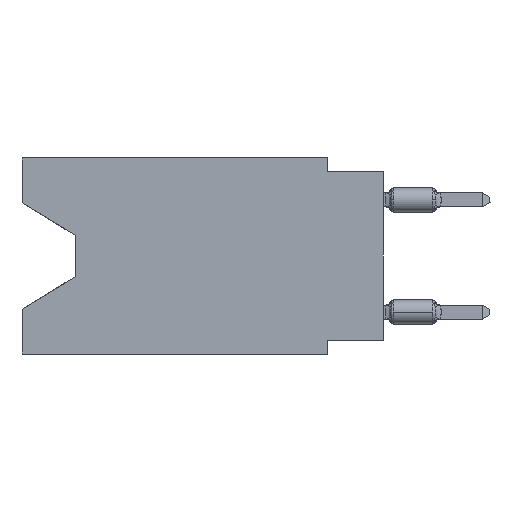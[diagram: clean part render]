
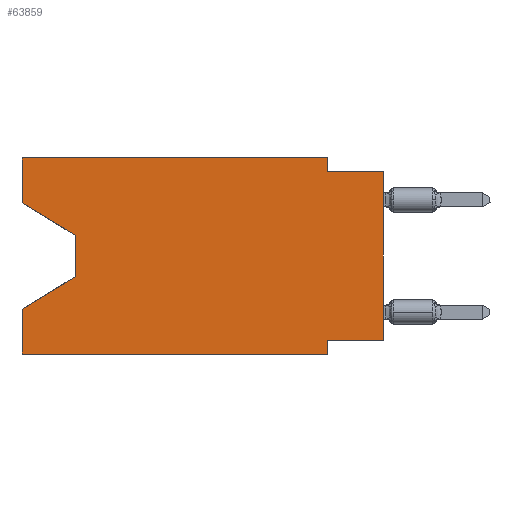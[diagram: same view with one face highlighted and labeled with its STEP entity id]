
A CAD part, left-side view. The second image highlights one B-rep face of the part: STEP entity #63859.
In plain terms, the highlighted planar face has unit normal (-1, 0, 0).
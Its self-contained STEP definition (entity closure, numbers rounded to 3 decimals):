
#559 = CARTESIAN_POINT ( 'NONE',  ( 0., 16.383, 0. ) ) ;
#798 = DIRECTION ( 'NONE',  ( 0., 1., 0. ) ) ;
#1833 = CARTESIAN_POINT ( 'NONE',  ( 0., 16.383, -8.89 ) ) ;
#2455 = VERTEX_POINT ( 'NONE', #49989 ) ;
#4818 = EDGE_CURVE ( 'NONE', #67629, #2455, #16789, .T. ) ;
#5903 = VECTOR ( 'NONE', #16608, 1000. ) ;
#6287 = VECTOR ( 'NONE', #33199, 1000. ) ;
#6741 = EDGE_CURVE ( 'NONE', #42762, #55426, #18316, .T. ) ;
#9593 = LINE ( 'NONE', #45181, #66337 ) ;
#9810 = DIRECTION ( 'NONE',  ( 0., -1., 0. ) ) ;
#10538 = VERTEX_POINT ( 'NONE', #1833 ) ;
#10824 = LINE ( 'NONE', #31768, #51969 ) ;
#13276 = CARTESIAN_POINT ( 'NONE',  ( 0., 16.383, -2.038 ) ) ;
#13336 = VECTOR ( 'NONE', #17821, 1000. ) ;
#13357 = ORIENTED_EDGE ( 'NONE', *, *, #4818, .T. ) ;
#13374 = LINE ( 'NONE', #45108, #52631 ) ;
#13657 = EDGE_LOOP ( 'NONE', ( #64866, #23779, #13357, #47135, #57510, #18241, #57631, #34532, #55323, #53581, #33526, #62559 ) ) ;
#16271 = CARTESIAN_POINT ( 'NONE',  ( 0., 13.97, -3.505 ) ) ;
#16608 = DIRECTION ( 'NONE',  ( 0., 0., 1. ) ) ;
#16789 = LINE ( 'NONE', #22018, #13336 ) ;
#17290 = CARTESIAN_POINT ( 'NONE',  ( 0., 13.97, -5.385 ) ) ;
#17821 = DIRECTION ( 'NONE',  ( 0., 0.855, -0.519 ) ) ;
#18241 = ORIENTED_EDGE ( 'NONE', *, *, #68927, .F. ) ;
#18316 = LINE ( 'NONE', #38890, #57024 ) ;
#18526 = LINE ( 'NONE', #13276, #6287 ) ;
#18632 = DIRECTION ( 'NONE',  ( 0., 0., -1. ) ) ;
#19743 = LINE ( 'NONE', #36111, #25132 ) ;
#20969 = DIRECTION ( 'NONE',  ( 0., 0., 1. ) ) ;
#21342 = LINE ( 'NONE', #42579, #40229 ) ;
#22018 = CARTESIAN_POINT ( 'NONE',  ( 0., 13.97, -5.385 ) ) ;
#23779 = ORIENTED_EDGE ( 'NONE', *, *, #60711, .T. ) ;
#23860 = DIRECTION ( 'NONE',  ( 0., -1., 0. ) ) ;
#24465 = VERTEX_POINT ( 'NONE', #47426 ) ;
#24531 = LINE ( 'NONE', #29422, #46024 ) ;
#25132 = VECTOR ( 'NONE', #45865, 1000. ) ;
#25624 = EDGE_CURVE ( 'NONE', #47585, #42762, #10824, .T. ) ;
#26387 = VERTEX_POINT ( 'NONE', #26996 ) ;
#26996 = CARTESIAN_POINT ( 'NONE',  ( 0., 2.54, -8.255 ) ) ;
#29287 = EDGE_CURVE ( 'NONE', #10538, #54925, #19743, .T. ) ;
#29293 = EDGE_CURVE ( 'NONE', #24465, #31701, #9593, .T. ) ;
#29422 = CARTESIAN_POINT ( 'NONE',  ( 0., 2.54, 0. ) ) ;
#30089 = EDGE_CURVE ( 'NONE', #47585, #36011, #18526, .T. ) ;
#30134 = DIRECTION ( 'NONE',  ( 0., 0., -1. ) ) ;
#30615 = DIRECTION ( 'NONE',  ( 1., 0., 0. ) ) ;
#31701 = VERTEX_POINT ( 'NONE', #54709 ) ;
#31768 = CARTESIAN_POINT ( 'NONE',  ( 0., 16.383, 0. ) ) ;
#32199 = CARTESIAN_POINT ( 'NONE',  ( 0., 0., -8.255 ) ) ;
#33199 = DIRECTION ( 'NONE',  ( 0., -0.855, -0.519 ) ) ;
#33526 = ORIENTED_EDGE ( 'NONE', *, *, #6741, .F. ) ;
#34532 = ORIENTED_EDGE ( 'NONE', *, *, #29293, .T. ) ;
#36011 = VERTEX_POINT ( 'NONE', #16271 ) ;
#36111 = CARTESIAN_POINT ( 'NONE',  ( 0., 16.383, -8.89 ) ) ;
#36189 = PLANE ( 'NONE',  #62425 ) ;
#37348 = CARTESIAN_POINT ( 'NONE',  ( 0., 2.54, -0.635 ) ) ;
#38006 = EDGE_CURVE ( 'NONE', #68493, #31701, #21342, .T. ) ;
#38890 = CARTESIAN_POINT ( 'NONE',  ( 0., 16.383, 0. ) ) ;
#39905 = LINE ( 'NONE', #67084, #63762 ) ;
#40229 = VECTOR ( 'NONE', #9810, 1000. ) ;
#41074 = FACE_OUTER_BOUND ( 'NONE', #13657, .T. ) ;
#41109 = EDGE_CURVE ( 'NONE', #24465, #26387, #54124, .T. ) ;
#42067 = LINE ( 'NONE', #559, #5903 ) ;
#42103 = CARTESIAN_POINT ( 'NONE',  ( 0., 16.383, 0. ) ) ;
#42579 = CARTESIAN_POINT ( 'NONE',  ( 0., 0., -0.635 ) ) ;
#42762 = VERTEX_POINT ( 'NONE', #50419 ) ;
#44438 = VECTOR ( 'NONE', #798, 1000. ) ;
#45108 = CARTESIAN_POINT ( 'NONE',  ( 0., 13.97, -3.505 ) ) ;
#45181 = CARTESIAN_POINT ( 'NONE',  ( 0., 0., 0. ) ) ;
#45865 = DIRECTION ( 'NONE',  ( 0., -1., 0. ) ) ;
#46024 = VECTOR ( 'NONE', #50686, 1000. ) ;
#47135 = ORIENTED_EDGE ( 'NONE', *, *, #68670, .F. ) ;
#47426 = CARTESIAN_POINT ( 'NONE',  ( 0., 0., -8.255 ) ) ;
#47585 = VERTEX_POINT ( 'NONE', #62664 ) ;
#47637 = CARTESIAN_POINT ( 'NONE',  ( 0., 2.54, 0. ) ) ;
#49989 = CARTESIAN_POINT ( 'NONE',  ( 0., 16.383, -6.852 ) ) ;
#50419 = CARTESIAN_POINT ( 'NONE',  ( 0., 16.383, 0. ) ) ;
#50686 = DIRECTION ( 'NONE',  ( 0., 0., -1. ) ) ;
#51865 = DIRECTION ( 'NONE',  ( 0., 0., -1. ) ) ;
#51969 = VECTOR ( 'NONE', #20969, 1000. ) ;
#52339 = EDGE_CURVE ( 'NONE', #55426, #68493, #24531, .T. ) ;
#52631 = VECTOR ( 'NONE', #18632, 1000. ) ;
#53581 = ORIENTED_EDGE ( 'NONE', *, *, #52339, .F. ) ;
#54124 = LINE ( 'NONE', #32199, #44438 ) ;
#54709 = CARTESIAN_POINT ( 'NONE',  ( 0., 0., -0.635 ) ) ;
#54925 = VERTEX_POINT ( 'NONE', #63048 ) ;
#55323 = ORIENTED_EDGE ( 'NONE', *, *, #38006, .F. ) ;
#55426 = VERTEX_POINT ( 'NONE', #47637 ) ;
#57024 = VECTOR ( 'NONE', #23860, 1000. ) ;
#57510 = ORIENTED_EDGE ( 'NONE', *, *, #29287, .T. ) ;
#57631 = ORIENTED_EDGE ( 'NONE', *, *, #41109, .F. ) ;
#60711 = EDGE_CURVE ( 'NONE', #36011, #67629, #13374, .T. ) ;
#62425 = AXIS2_PLACEMENT_3D ( 'NONE', #42103, #30615, #51865 ) ;
#62559 = ORIENTED_EDGE ( 'NONE', *, *, #25624, .F. ) ;
#62576 = DIRECTION ( 'NONE',  ( 0., 0., 1. ) ) ;
#62664 = CARTESIAN_POINT ( 'NONE',  ( 0., 16.383, -2.038 ) ) ;
#63048 = CARTESIAN_POINT ( 'NONE',  ( 0., 2.54, -8.89 ) ) ;
#63762 = VECTOR ( 'NONE', #30134, 1000. ) ;
#63859 = ADVANCED_FACE ( 'NONE', ( #41074 ), #36189, .F. ) ;
#64866 = ORIENTED_EDGE ( 'NONE', *, *, #30089, .T. ) ;
#66337 = VECTOR ( 'NONE', #62576, 1000. ) ;
#67084 = CARTESIAN_POINT ( 'NONE',  ( 0., 2.54, -8.89 ) ) ;
#67629 = VERTEX_POINT ( 'NONE', #17290 ) ;
#68493 = VERTEX_POINT ( 'NONE', #37348 ) ;
#68670 = EDGE_CURVE ( 'NONE', #10538, #2455, #42067, .T. ) ;
#68927 = EDGE_CURVE ( 'NONE', #26387, #54925, #39905, .T. ) ;
